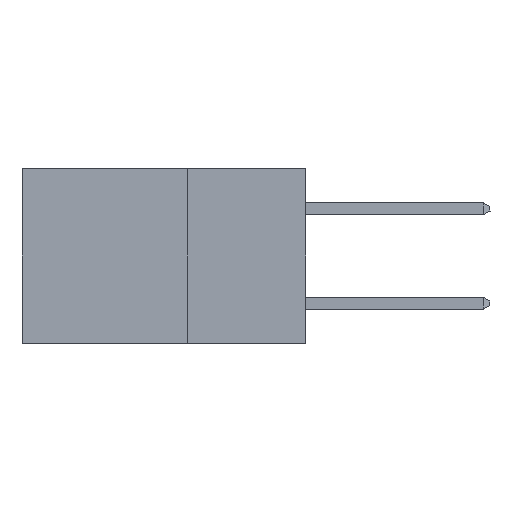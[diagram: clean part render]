
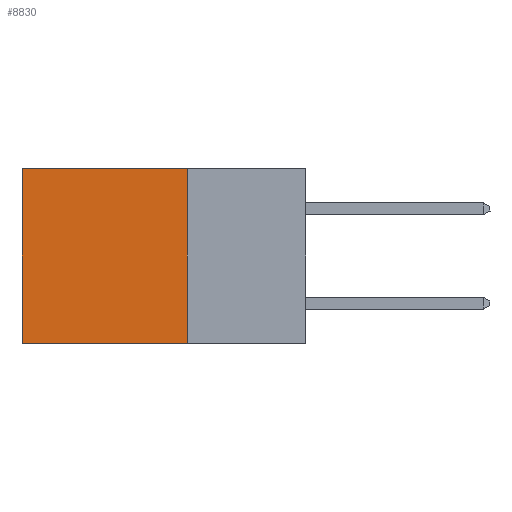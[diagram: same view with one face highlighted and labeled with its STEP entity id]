
A CAD part, left-side view. The second image highlights one B-rep face of the part: STEP entity #8830.
In plain terms, the highlighted planar face has unit normal (-1, 0, 0).
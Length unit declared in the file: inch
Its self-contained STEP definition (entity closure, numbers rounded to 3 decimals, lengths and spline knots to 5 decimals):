
#324 = DIRECTION ( 'NONE',  ( 0., 1., 0. ) ) ;
#368 = CARTESIAN_POINT ( 'NONE',  ( 0.298, 0.6, -0.37 ) ) ;
#438 = CARTESIAN_POINT ( 'NONE',  ( 0.298, 0.6, 0. ) ) ;
#577 = DIRECTION ( 'NONE',  ( 0., 0., -1. ) ) ;
#650 = CARTESIAN_POINT ( 'NONE',  ( 0.298, 0.6, 0. ) ) ;
#901 = DIRECTION ( 'NONE',  ( 0., 0., -1. ) ) ;
#1397 = PLANE ( 'NONE',  #6074 ) ;
#1582 = VERTEX_POINT ( 'NONE', #3637 ) ;
#1774 = CARTESIAN_POINT ( 'NONE',  ( 0.298, 0.25, 0. ) ) ;
#2281 = ORIENTED_EDGE ( 'NONE', *, *, #6902, .T. ) ;
#2370 = VERTEX_POINT ( 'NONE', #368 ) ;
#2425 = VECTOR ( 'NONE', #577, 39.37008 ) ;
#2972 = CARTESIAN_POINT ( 'NONE',  ( 0.298, 0.25, 0. ) ) ;
#3637 = CARTESIAN_POINT ( 'NONE',  ( 0.298, 0.25, -0.37 ) ) ;
#3656 = VECTOR ( 'NONE', #4429, 39.37008 ) ;
#3836 = DIRECTION ( 'NONE',  ( 1., 0., 0. ) ) ;
#4112 = EDGE_LOOP ( 'NONE', ( #5578, #5090, #4543, #2281 ) ) ;
#4150 = LINE ( 'NONE', #4460, #3656 ) ;
#4429 = DIRECTION ( 'NONE',  ( 0., 1., 0. ) ) ;
#4460 = CARTESIAN_POINT ( 'NONE',  ( 0.298, 0.25, -0.37 ) ) ;
#4543 = ORIENTED_EDGE ( 'NONE', *, *, #8441, .F. ) ;
#5090 = ORIENTED_EDGE ( 'NONE', *, *, #8216, .F. ) ;
#5396 = DIRECTION ( 'NONE',  ( 0., 0., -1. ) ) ;
#5506 = VECTOR ( 'NONE', #901, 39.37008 ) ;
#5578 = ORIENTED_EDGE ( 'NONE', *, *, #8222, .T. ) ;
#5624 = FACE_OUTER_BOUND ( 'NONE', #4112, .T. ) ;
#6074 = AXIS2_PLACEMENT_3D ( 'NONE', #2972, #3836, #5396 ) ;
#6491 = VERTEX_POINT ( 'NONE', #650 ) ;
#6902 = EDGE_CURVE ( 'NONE', #7604, #6491, #9638, .T. ) ;
#7604 = VERTEX_POINT ( 'NONE', #1774 ) ;
#7771 = CARTESIAN_POINT ( 'NONE',  ( 0.298, 0.25, 0. ) ) ;
#8185 = LINE ( 'NONE', #7771, #5506 ) ;
#8216 = EDGE_CURVE ( 'NONE', #1582, #2370, #4150, .T. ) ;
#8222 = EDGE_CURVE ( 'NONE', #6491, #2370, #9359, .T. ) ;
#8441 = EDGE_CURVE ( 'NONE', #7604, #1582, #8185, .T. ) ;
#8787 = CARTESIAN_POINT ( 'NONE',  ( 0.298, 0.25, 0. ) ) ;
#8830 = ADVANCED_FACE ( 'NONE', ( #5624 ), #1397, .F. ) ;
#9359 = LINE ( 'NONE', #438, #2425 ) ;
#9393 = VECTOR ( 'NONE', #324, 39.37008 ) ;
#9638 = LINE ( 'NONE', #8787, #9393 ) ;
